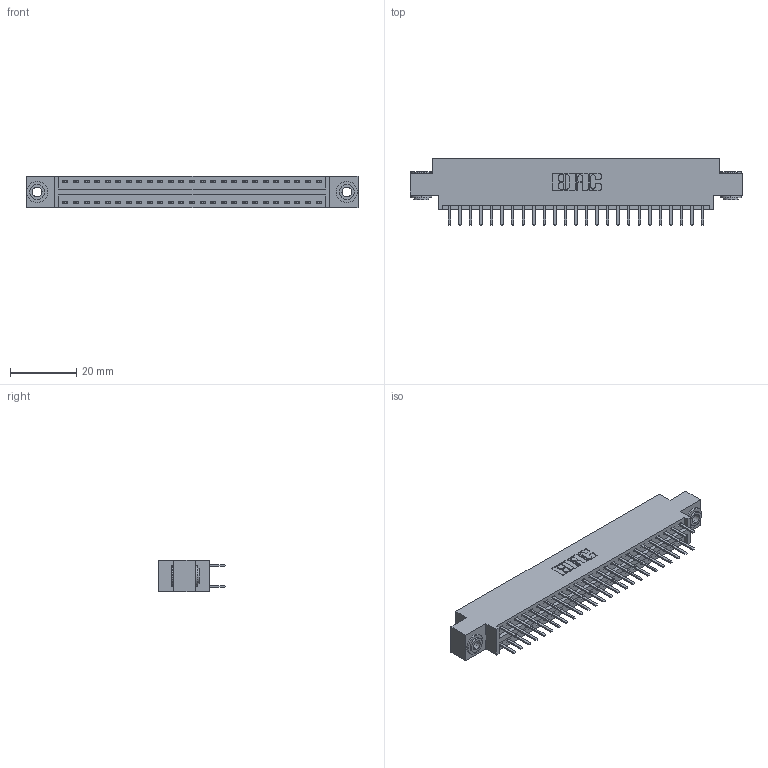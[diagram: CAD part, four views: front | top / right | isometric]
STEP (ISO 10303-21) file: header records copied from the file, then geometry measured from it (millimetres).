
FILE_DESCRIPTION (( 'STEP AP203' ), '1' );
FILE_NAME ('396-050-520-803.STEP', '2019-11-02T07:11:41', ( '' ), ( '' ), 'SwSTEP 2.0', 'SolidWorks 2016', '' );
FILE_SCHEMA (( 'CONFIG_CONTROL_DESIGN' ));
Length unit declared in the file: inch
Products named in the file (4): 346 Part_0.170 Offset - 0.156 Dia-TH; 345-292-001_345-293-120; 345-250-002_345-250-002-102; 396-050-520-803
Assembly tree (53 placements, depth 2):
  396-050-520-803
    346 Part_0.170 Offset - 0.156 Dia-TH
    345-292-001_345-293-120  x50
    345-250-002_345-250-002-102  x2
Bounding box: 99.95 x 20.02 x 9.4 mm (x, y, z)
Volume: 9457 mm3; surface area: 13074.4 mm2
Topology: 53 solids, 53 shells, 2964 faces, 8567 edges, 5574 vertices
Faces by surface type: plane 1940, cylinder 1016, cone 8
Entity records: 19500 total; most frequent: CARTESIAN_POINT 3227, ORIENTED_EDGE 3142, DIRECTION 2913, EDGE_CURVE 1571, LINE 1311, VECTOR 1311, VERTEX_POINT 1042, AXIS2_PLACEMENT_3D 801
